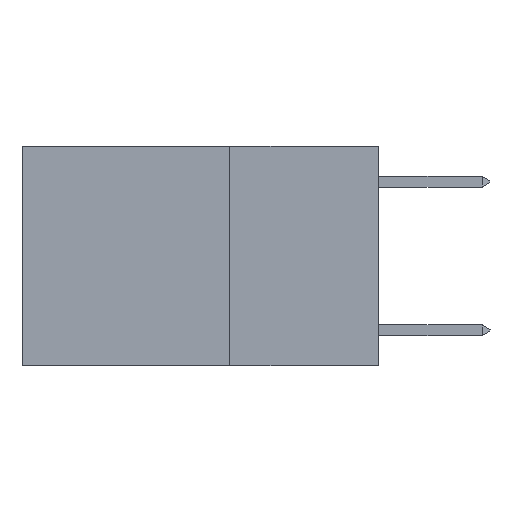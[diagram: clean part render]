
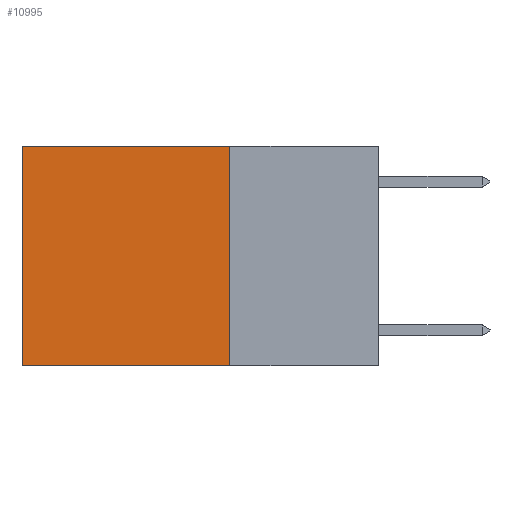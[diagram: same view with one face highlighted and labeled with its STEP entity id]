
A CAD part, left-side view. The second image highlights one B-rep face of the part: STEP entity #10995.
In plain terms, the highlighted planar face has unit normal (-1, 0, 0).
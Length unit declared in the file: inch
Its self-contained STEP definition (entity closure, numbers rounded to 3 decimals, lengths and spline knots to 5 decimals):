
#390 = DIRECTION ( 'NONE',  ( 1., 0., 0. ) ) ;
#1143 = CARTESIAN_POINT ( 'NONE',  ( 0.2625, 0.25, 0. ) ) ;
#1175 = ORIENTED_EDGE ( 'NONE', *, *, #2746, .T. ) ;
#1922 = VERTEX_POINT ( 'NONE', #3634 ) ;
#1998 = LINE ( 'NONE', #11642, #12511 ) ;
#2746 = EDGE_CURVE ( 'NONE', #3571, #11911, #3784, .T. ) ;
#2856 = EDGE_CURVE ( 'NONE', #11911, #1922, #1998, .T. ) ;
#2924 = CARTESIAN_POINT ( 'NONE',  ( 0.2625, 0.25, 0. ) ) ;
#3023 = CARTESIAN_POINT ( 'NONE',  ( 0.2625, 0.6, 0. ) ) ;
#3404 = ORIENTED_EDGE ( 'NONE', *, *, #7748, .F. ) ;
#3421 = AXIS2_PLACEMENT_3D ( 'NONE', #9265, #390, #8314 ) ;
#3571 = VERTEX_POINT ( 'NONE', #9797 ) ;
#3634 = CARTESIAN_POINT ( 'NONE',  ( 0.2625, 0.6, -0.37 ) ) ;
#3784 = LINE ( 'NONE', #2924, #5990 ) ;
#5318 = VERTEX_POINT ( 'NONE', #6147 ) ;
#5525 = CARTESIAN_POINT ( 'NONE',  ( 0.2625, 0.25, -0.37 ) ) ;
#5990 = VECTOR ( 'NONE', #7221, 39.37008 ) ;
#6147 = CARTESIAN_POINT ( 'NONE',  ( 0.2625, 0.25, -0.37 ) ) ;
#6270 = PLANE ( 'NONE',  #3421 ) ;
#7221 = DIRECTION ( 'NONE',  ( 0., 1., 0. ) ) ;
#7575 = DIRECTION ( 'NONE',  ( 0., 1., 0. ) ) ;
#7748 = EDGE_CURVE ( 'NONE', #3571, #5318, #12283, .T. ) ;
#8139 = DIRECTION ( 'NONE',  ( 0., 0., -1. ) ) ;
#8203 = LINE ( 'NONE', #5525, #9646 ) ;
#8314 = DIRECTION ( 'NONE',  ( 0., 0., -1. ) ) ;
#8947 = EDGE_LOOP ( 'NONE', ( #11155, #9580, #3404, #1175 ) ) ;
#9265 = CARTESIAN_POINT ( 'NONE',  ( 0.2625, 0.25, 0. ) ) ;
#9580 = ORIENTED_EDGE ( 'NONE', *, *, #12747, .F. ) ;
#9646 = VECTOR ( 'NONE', #7575, 39.37008 ) ;
#9797 = CARTESIAN_POINT ( 'NONE',  ( 0.2625, 0.25, 0. ) ) ;
#10995 = ADVANCED_FACE ( 'NONE', ( #11254 ), #6270, .F. ) ;
#11155 = ORIENTED_EDGE ( 'NONE', *, *, #2856, .T. ) ;
#11254 = FACE_OUTER_BOUND ( 'NONE', #8947, .T. ) ;
#11642 = CARTESIAN_POINT ( 'NONE',  ( 0.2625, 0.6, 0. ) ) ;
#11773 = DIRECTION ( 'NONE',  ( 0., 0., -1. ) ) ;
#11911 = VERTEX_POINT ( 'NONE', #3023 ) ;
#12283 = LINE ( 'NONE', #1143, #12936 ) ;
#12511 = VECTOR ( 'NONE', #11773, 39.37008 ) ;
#12747 = EDGE_CURVE ( 'NONE', #5318, #1922, #8203, .T. ) ;
#12936 = VECTOR ( 'NONE', #8139, 39.37008 ) ;
